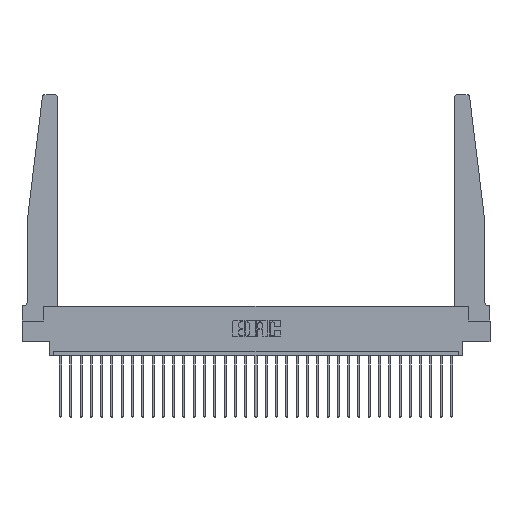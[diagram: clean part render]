
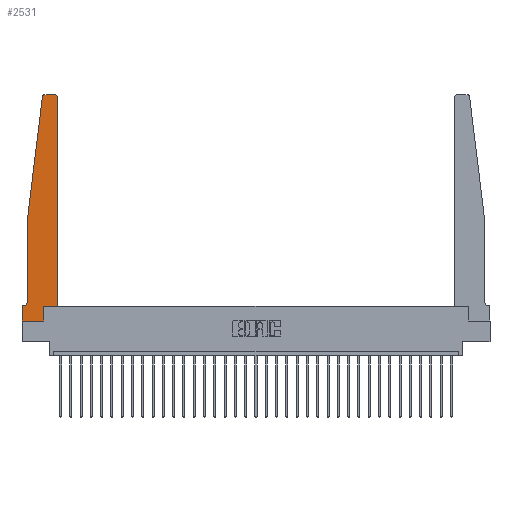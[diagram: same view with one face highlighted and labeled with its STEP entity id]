
A CAD part, top view. The second image highlights one B-rep face of the part: STEP entity #2531.
In plain terms, the highlighted planar face has unit normal (0, 0, 1).
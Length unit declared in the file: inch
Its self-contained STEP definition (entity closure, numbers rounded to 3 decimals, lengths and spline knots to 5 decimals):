
#182 = EDGE_CURVE ( 'NONE', #19500, #2852, #1024, .T. ) ;
#579 = ORIENTED_EDGE ( 'NONE', *, *, #16921, .T. ) ;
#907 = ORIENTED_EDGE ( 'NONE', *, *, #28274, .T. ) ;
#1024 = LINE ( 'NONE', #5410, #5704 ) ;
#1034 = CARTESIAN_POINT ( 'NONE',  ( 0., 0., 0.37 ) ) ;
#1314 = CARTESIAN_POINT ( 'NONE',  ( 0.065, 1.25, 0.37 ) ) ;
#1798 = LINE ( 'NONE', #17838, #8435 ) ;
#1802 = VERTEX_POINT ( 'NONE', #2983 ) ;
#2100 = DIRECTION ( 'NONE',  ( 0., 1., 0. ) ) ;
#2470 = AXIS2_PLACEMENT_3D ( 'NONE', #12545, #3750, #10401 ) ;
#2531 = ADVANCED_FACE ( 'NONE', ( #21087 ), #24050, .T. ) ;
#2852 = VERTEX_POINT ( 'NONE', #18622 ) ;
#2983 = CARTESIAN_POINT ( 'NONE',  ( 0.065, 0.2375, 0.37 ) ) ;
#3112 = CIRCLE ( 'NONE', #7460, 0.03 ) ;
#3594 = ORIENTED_EDGE ( 'NONE', *, *, #12250, .T. ) ;
#3730 = DIRECTION ( 'NONE',  ( -0.122, -0.992, 0. ) ) ;
#3750 = DIRECTION ( 'NONE',  ( 0., 0., -1. ) ) ;
#3881 = ORIENTED_EDGE ( 'NONE', *, *, #18974, .T. ) ;
#4489 = ORIENTED_EDGE ( 'NONE', *, *, #182, .T. ) ;
#4491 = VERTEX_POINT ( 'NONE', #6213 ) ;
#5005 = EDGE_CURVE ( 'NONE', #11720, #26914, #21513, .T. ) ;
#5410 = CARTESIAN_POINT ( 'NONE',  ( 0.25, 2.75, 0.37 ) ) ;
#5620 = DIRECTION ( 'NONE',  ( 1., 0., 0. ) ) ;
#5704 = VECTOR ( 'NONE', #14650, 39.37008 ) ;
#6029 = LINE ( 'NONE', #1034, #20411 ) ;
#6213 = CARTESIAN_POINT ( 'NONE',  ( 0.015, 0.1875, 0.37 ) ) ;
#6567 = EDGE_CURVE ( 'NONE', #1802, #4491, #9247, .T. ) ;
#6836 = CARTESIAN_POINT ( 'NONE',  ( 0.2605, 0.18, 0.37 ) ) ;
#6980 = VECTOR ( 'NONE', #7635, 39.37008 ) ;
#7034 = VECTOR ( 'NONE', #3730, 39.37008 ) ;
#7460 = AXIS2_PLACEMENT_3D ( 'NONE', #17132, #28504, #5620 ) ;
#7635 = DIRECTION ( 'NONE',  ( 1., 0., 0. ) ) ;
#7696 = EDGE_CURVE ( 'NONE', #4491, #15657, #9669, .T. ) ;
#7983 = EDGE_CURVE ( 'NONE', #15657, #11720, #6029, .T. ) ;
#8104 = EDGE_LOOP ( 'NONE', ( #4489, #21548, #16494, #907, #25388, #29913, #20026, #21868, #24091, #579, #3594, #3881 ) ) ;
#8435 = VECTOR ( 'NONE', #2100, 39.37008 ) ;
#8974 = DIRECTION ( 'NONE',  ( 0., -1., 0. ) ) ;
#9011 = VECTOR ( 'NONE', #8974, 39.37008 ) ;
#9102 = VERTEX_POINT ( 'NONE', #11682 ) ;
#9126 = LINE ( 'NONE', #16378, #9011 ) ;
#9247 = CIRCLE ( 'NONE', #2470, 0.05 ) ;
#9669 = LINE ( 'NONE', #23443, #10201 ) ;
#10201 = VECTOR ( 'NONE', #16361, 39.37008 ) ;
#10401 = DIRECTION ( 'NONE',  ( -1., 0., 0. ) ) ;
#11037 = LINE ( 'NONE', #26951, #28712 ) ;
#11471 = AXIS2_PLACEMENT_3D ( 'NONE', #13582, #17970, #16155 ) ;
#11682 = CARTESIAN_POINT ( 'NONE',  ( 0.24675, 2.72367, 0.37 ) ) ;
#11720 = VERTEX_POINT ( 'NONE', #17876 ) ;
#12250 = EDGE_CURVE ( 'NONE', #28540, #15302, #1798, .T. ) ;
#12545 = CARTESIAN_POINT ( 'NONE',  ( 0.015, 0.2375, 0.37 ) ) ;
#13582 = CARTESIAN_POINT ( 'NONE',  ( 0.27653, 2.72, 0.37 ) ) ;
#13586 = EDGE_CURVE ( 'NONE', #9102, #25813, #26608, .T. ) ;
#13924 = CARTESIAN_POINT ( 'NONE',  ( 0.395, 2.75, 0.37 ) ) ;
#14292 = DIRECTION ( 'NONE',  ( 1., 0., 0. ) ) ;
#14351 = CARTESIAN_POINT ( 'NONE',  ( 0.2605, 0., 0.37 ) ) ;
#14570 = VECTOR ( 'NONE', #19570, 39.37008 ) ;
#14650 = DIRECTION ( 'NONE',  ( -1., 0., 0. ) ) ;
#15008 = AXIS2_PLACEMENT_3D ( 'NONE', #28638, #28063, #14292 ) ;
#15073 = CARTESIAN_POINT ( 'NONE',  ( 0.065, 1.25, 0.37 ) ) ;
#15302 = VERTEX_POINT ( 'NONE', #17785 ) ;
#15657 = VERTEX_POINT ( 'NONE', #28820 ) ;
#16155 = DIRECTION ( 'NONE',  ( 1., 0., 0. ) ) ;
#16361 = DIRECTION ( 'NONE',  ( -1., 0., 0. ) ) ;
#16378 = CARTESIAN_POINT ( 'NONE',  ( 0.065, 1.25, 0.37 ) ) ;
#16494 = ORIENTED_EDGE ( 'NONE', *, *, #13586, .T. ) ;
#16921 = EDGE_CURVE ( 'NONE', #19944, #28540, #28865, .T. ) ;
#17132 = CARTESIAN_POINT ( 'NONE',  ( 0.395, 2.72, 0.37 ) ) ;
#17785 = CARTESIAN_POINT ( 'NONE',  ( 0.425, 2.72, 0.37 ) ) ;
#17838 = CARTESIAN_POINT ( 'NONE',  ( 0.425, 0.18, 0.37 ) ) ;
#17876 = CARTESIAN_POINT ( 'NONE',  ( 0., 0., 0.37 ) ) ;
#17970 = DIRECTION ( 'NONE',  ( 0., 0., 1. ) ) ;
#18622 = CARTESIAN_POINT ( 'NONE',  ( 0.27653, 2.75, 0.37 ) ) ;
#18974 = EDGE_CURVE ( 'NONE', #15302, #19500, #3112, .T. ) ;
#19017 = CARTESIAN_POINT ( 'NONE',  ( 0.425, 0.18, 0.37 ) ) ;
#19500 = VERTEX_POINT ( 'NONE', #13924 ) ;
#19570 = DIRECTION ( 'NONE',  ( 1., 0., 0. ) ) ;
#19944 = VERTEX_POINT ( 'NONE', #6836 ) ;
#20026 = ORIENTED_EDGE ( 'NONE', *, *, #7983, .T. ) ;
#20265 = DIRECTION ( 'NONE',  ( 0., 1., 0. ) ) ;
#20411 = VECTOR ( 'NONE', #26943, 39.37008 ) ;
#21087 = FACE_OUTER_BOUND ( 'NONE', #8104, .T. ) ;
#21513 = LINE ( 'NONE', #26395, #14570 ) ;
#21548 = ORIENTED_EDGE ( 'NONE', *, *, #29567, .T. ) ;
#21868 = ORIENTED_EDGE ( 'NONE', *, *, #5005, .T. ) ;
#22542 = CIRCLE ( 'NONE', #11471, 0.03 ) ;
#23443 = CARTESIAN_POINT ( 'NONE',  ( 0.065, 0.1875, 0.37 ) ) ;
#24050 = PLANE ( 'NONE',  #15008 ) ;
#24091 = ORIENTED_EDGE ( 'NONE', *, *, #25580, .T. ) ;
#25388 = ORIENTED_EDGE ( 'NONE', *, *, #6567, .T. ) ;
#25580 = EDGE_CURVE ( 'NONE', #26914, #19944, #11037, .T. ) ;
#25813 = VERTEX_POINT ( 'NONE', #1314 ) ;
#26395 = CARTESIAN_POINT ( 'NONE',  ( 0., 0., 0.37 ) ) ;
#26608 = LINE ( 'NONE', #15073, #7034 ) ;
#26645 = CARTESIAN_POINT ( 'NONE',  ( 0.425, 0.18, 0.37 ) ) ;
#26914 = VERTEX_POINT ( 'NONE', #14351 ) ;
#26943 = DIRECTION ( 'NONE',  ( 0., -1., 0. ) ) ;
#26951 = CARTESIAN_POINT ( 'NONE',  ( 0.2605, 0.18, 0.37 ) ) ;
#28063 = DIRECTION ( 'NONE',  ( 0., 0., 1. ) ) ;
#28274 = EDGE_CURVE ( 'NONE', #25813, #1802, #9126, .T. ) ;
#28504 = DIRECTION ( 'NONE',  ( 0., 0., 1. ) ) ;
#28540 = VERTEX_POINT ( 'NONE', #26645 ) ;
#28638 = CARTESIAN_POINT ( 'NONE',  ( 0., 0.1875, 0.37 ) ) ;
#28712 = VECTOR ( 'NONE', #20265, 39.37008 ) ;
#28820 = CARTESIAN_POINT ( 'NONE',  ( 0., 0.1875, 0.37 ) ) ;
#28865 = LINE ( 'NONE', #19017, #6980 ) ;
#29567 = EDGE_CURVE ( 'NONE', #2852, #9102, #22542, .T. ) ;
#29913 = ORIENTED_EDGE ( 'NONE', *, *, #7696, .T. ) ;
